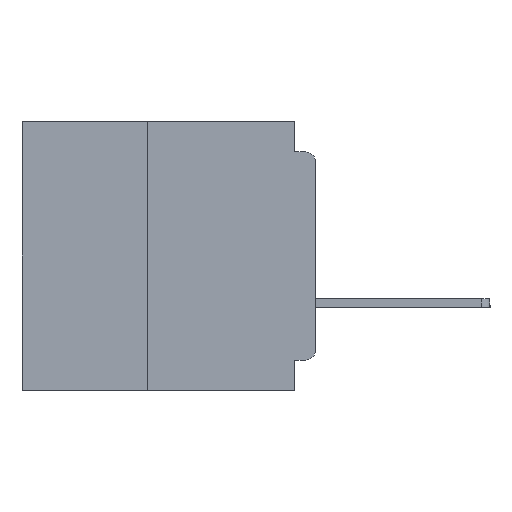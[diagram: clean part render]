
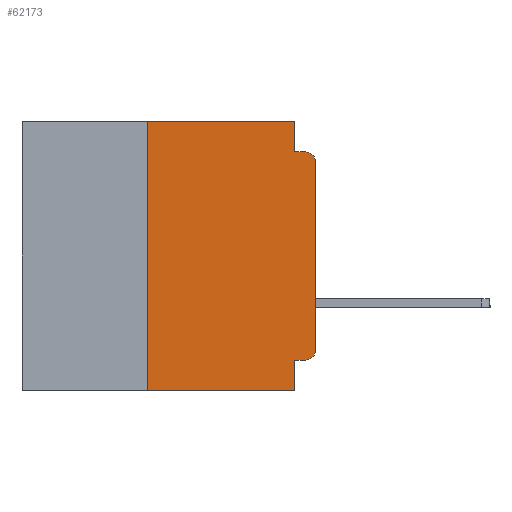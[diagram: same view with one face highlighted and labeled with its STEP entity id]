
A CAD part, left-side view. The second image highlights one B-rep face of the part: STEP entity #62173.
In plain terms, the highlighted planar face has unit normal (-1, 0, 0).
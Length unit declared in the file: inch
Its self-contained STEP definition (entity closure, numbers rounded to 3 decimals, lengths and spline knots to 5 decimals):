
#62 = VECTOR ( 'NONE', #14063, 39.37008 ) ;
#1510 = CARTESIAN_POINT ( 'NONE',  ( 0., 0., 0. ) ) ;
#1582 = FACE_OUTER_BOUND ( 'NONE', #5054, .T. ) ;
#2369 = CARTESIAN_POINT ( 'NONE',  ( 0., 0., -0.045 ) ) ;
#2873 = VECTOR ( 'NONE', #63187, 39.37008 ) ;
#3282 = LINE ( 'NONE', #39802, #62 ) ;
#3925 = DIRECTION ( 'NONE',  ( 1., 0., 0. ) ) ;
#4856 = ORIENTED_EDGE ( 'NONE', *, *, #52799, .F. ) ;
#5054 = EDGE_LOOP ( 'NONE', ( #13793, #39380, #4856, #37691, #5660, #9895, #43543, #37556, #44831, #9445 ) ) ;
#5333 = EDGE_CURVE ( 'NONE', #21896, #45558, #21801, .T. ) ;
#5660 = ORIENTED_EDGE ( 'NONE', *, *, #5333, .F. ) ;
#6670 = EDGE_CURVE ( 'NONE', #38248, #21896, #9561, .T. ) ;
#6669 = DIRECTION ( 'NONE',  ( 0., 0., 1. ) ) ;
#7920 = VECTOR ( 'NONE', #31788, 39.37008 ) ;
#8104 = VECTOR ( 'NONE', #14712, 39.37008 ) ;
#8876 = AXIS2_PLACEMENT_3D ( 'NONE', #19238, #3925, #40030 ) ;
#9445 = ORIENTED_EDGE ( 'NONE', *, *, #54421, .T. ) ;
#9561 = LINE ( 'NONE', #26577, #7920 ) ;
#9895 = ORIENTED_EDGE ( 'NONE', *, *, #6670, .F. ) ;
#10244 = CARTESIAN_POINT ( 'NONE',  ( 0., 0., -0.06 ) ) ;
#11038 = CIRCLE ( 'NONE', #14961, 0.015 ) ;
#12603 = VECTOR ( 'NONE', #6669, 39.37008 ) ;
#13668 = LINE ( 'NONE', #2369, #39529 ) ;
#13793 = ORIENTED_EDGE ( 'NONE', *, *, #33245, .T. ) ;
#13837 = DIRECTION ( 'NONE',  ( 0., -1., 0. ) ) ;
#14063 = DIRECTION ( 'NONE',  ( 0., 1., 0. ) ) ;
#14712 = DIRECTION ( 'NONE',  ( 0., -1., 0. ) ) ;
#14961 = AXIS2_PLACEMENT_3D ( 'NONE', #21518, #57446, #26766 ) ;
#16319 = VERTEX_POINT ( 'NONE', #60165 ) ;
#16511 = VERTEX_POINT ( 'NONE', #10244 ) ;
#17854 = DIRECTION ( 'NONE',  ( 0., -1., 0. ) ) ;
#19238 = CARTESIAN_POINT ( 'NONE',  ( 0., 0.437, 0. ) ) ;
#20910 = CARTESIAN_POINT ( 'NONE',  ( 0., 0.031, -0.4 ) ) ;
#21151 = CARTESIAN_POINT ( 'NONE',  ( 0., 0.031, -0.045 ) ) ;
#21518 = CARTESIAN_POINT ( 'NONE',  ( 0., 0.015, -0.34 ) ) ;
#21801 = LINE ( 'NONE', #24893, #8104 ) ;
#21896 = VERTEX_POINT ( 'NONE', #66449 ) ;
#24893 = CARTESIAN_POINT ( 'NONE',  ( 0., 0.437, 0. ) ) ;
#25395 = DIRECTION ( 'NONE',  ( -1., 0., 0. ) ) ;
#26577 = CARTESIAN_POINT ( 'NONE',  ( 0., 0.25, -0.4 ) ) ;
#26766 = DIRECTION ( 'NONE',  ( 0., 0., -1. ) ) ;
#27203 = CARTESIAN_POINT ( 'NONE',  ( 0., 0.031, -0.4 ) ) ;
#29224 = CARTESIAN_POINT ( 'NONE',  ( 0., 0.437, -0.4 ) ) ;
#29853 = VERTEX_POINT ( 'NONE', #64211 ) ;
#30246 = CARTESIAN_POINT ( 'NONE',  ( 0., 0.015, -0.045 ) ) ;
#31788 = DIRECTION ( 'NONE',  ( 0., 0., 1. ) ) ;
#32419 = EDGE_CURVE ( 'NONE', #38248, #66409, #50376, .T. ) ;
#32849 = LINE ( 'NONE', #27203, #40043 ) ;
#33245 = EDGE_CURVE ( 'NONE', #29853, #16511, #53622, .T. ) ;
#37556 = ORIENTED_EDGE ( 'NONE', *, *, #58760, .F. ) ;
#37691 = ORIENTED_EDGE ( 'NONE', *, *, #43457, .F. ) ;
#37697 = CARTESIAN_POINT ( 'NONE',  ( 0., 0.031, 0. ) ) ;
#38248 = VERTEX_POINT ( 'NONE', #64779 ) ;
#38511 = AXIS2_PLACEMENT_3D ( 'NONE', #56117, #25395, #61301 ) ;
#39380 = ORIENTED_EDGE ( 'NONE', *, *, #58545, .T. ) ;
#39529 = VECTOR ( 'NONE', #17854, 39.37008 ) ;
#39802 = CARTESIAN_POINT ( 'NONE',  ( 0., 0., -0.355 ) ) ;
#40030 = DIRECTION ( 'NONE',  ( 0., 0., -1. ) ) ;
#40043 = VECTOR ( 'NONE', #62843, 39.37008 ) ;
#40807 = LINE ( 'NONE', #37697, #2873 ) ;
#41911 = VERTEX_POINT ( 'NONE', #30246 ) ;
#43457 = EDGE_CURVE ( 'NONE', #45558, #53770, #40807, .T. ) ;
#43543 = ORIENTED_EDGE ( 'NONE', *, *, #32419, .T. ) ;
#44831 = ORIENTED_EDGE ( 'NONE', *, *, #47675, .F. ) ;
#45558 = VERTEX_POINT ( 'NONE', #49935 ) ;
#47675 = EDGE_CURVE ( 'NONE', #16319, #54794, #3282, .T. ) ;
#48815 = VECTOR ( 'NONE', #13837, 39.37008 ) ;
#49935 = CARTESIAN_POINT ( 'NONE',  ( 0., 0.031, 0. ) ) ;
#50059 = PLANE ( 'NONE',  #8876 ) ;
#50376 = LINE ( 'NONE', #29224, #48815 ) ;
#52799 = EDGE_CURVE ( 'NONE', #53770, #41911, #13668, .T. ) ;
#53622 = LINE ( 'NONE', #1510, #12603 ) ;
#53770 = VERTEX_POINT ( 'NONE', #21151 ) ;
#54421 = EDGE_CURVE ( 'NONE', #16319, #29853, #11038, .T. ) ;
#54794 = VERTEX_POINT ( 'NONE', #55168 ) ;
#55168 = CARTESIAN_POINT ( 'NONE',  ( 0., 0.031, -0.355 ) ) ;
#56117 = CARTESIAN_POINT ( 'NONE',  ( 0., 0.015, -0.06 ) ) ;
#57446 = DIRECTION ( 'NONE',  ( -1., 0., 0. ) ) ;
#57635 = CIRCLE ( 'NONE', #38511, 0.015 ) ;
#58545 = EDGE_CURVE ( 'NONE', #16511, #41911, #57635, .T. ) ;
#58760 = EDGE_CURVE ( 'NONE', #54794, #66409, #32849, .T. ) ;
#60165 = CARTESIAN_POINT ( 'NONE',  ( 0., 0.015, -0.355 ) ) ;
#61301 = DIRECTION ( 'NONE',  ( 0., 0., -1. ) ) ;
#62173 = ADVANCED_FACE ( 'NONE', ( #1582 ), #50059, .F. ) ;
#62843 = DIRECTION ( 'NONE',  ( 0., 0., -1. ) ) ;
#63187 = DIRECTION ( 'NONE',  ( 0., 0., -1. ) ) ;
#64211 = CARTESIAN_POINT ( 'NONE',  ( 0., 0., -0.34 ) ) ;
#64779 = CARTESIAN_POINT ( 'NONE',  ( 0., 0.25, -0.4 ) ) ;
#66409 = VERTEX_POINT ( 'NONE', #20910 ) ;
#66449 = CARTESIAN_POINT ( 'NONE',  ( 0., 0.25, 0. ) ) ;
